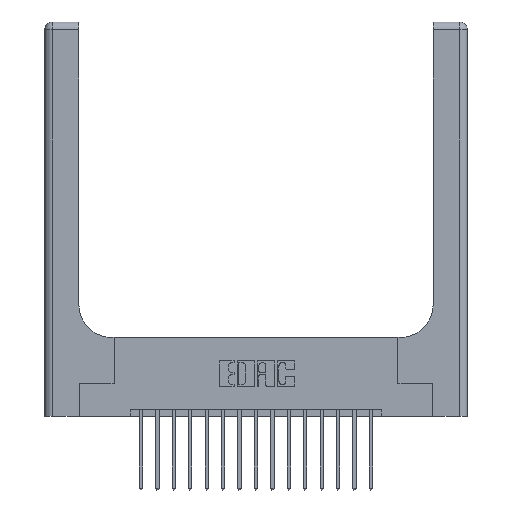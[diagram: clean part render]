
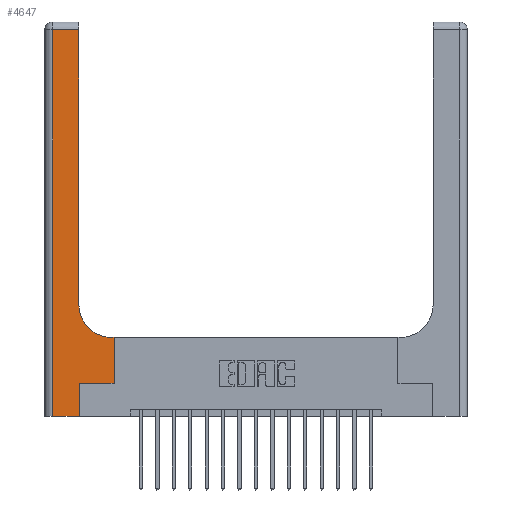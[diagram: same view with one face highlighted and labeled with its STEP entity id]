
A CAD part, top view. The second image highlights one B-rep face of the part: STEP entity #4647.
In plain terms, the highlighted planar face has unit normal (0, 0, 1).
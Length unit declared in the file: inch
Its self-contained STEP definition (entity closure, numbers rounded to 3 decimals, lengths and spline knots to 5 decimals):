
#137 = ORIENTED_EDGE ( 'NONE', *, *, #2642, .T. ) ;
#189 = PLANE ( 'NONE',  #9917 ) ;
#573 = VECTOR ( 'NONE', #8498, 39.37008 ) ;
#808 = VERTEX_POINT ( 'NONE', #2293 ) ;
#903 = CARTESIAN_POINT ( 'NONE',  ( 0.06, 0., 0.37 ) ) ;
#1154 = DIRECTION ( 'NONE',  ( -1., 0., 0. ) ) ;
#1228 = EDGE_CURVE ( 'NONE', #11090, #4433, #3883, .T. ) ;
#1326 = LINE ( 'NONE', #17534, #6257 ) ;
#1835 = DIRECTION ( 'NONE',  ( 0., 0., -1. ) ) ;
#1929 = CARTESIAN_POINT ( 'NONE',  ( 0., 3., 0.37 ) ) ;
#2078 = AXIS2_PLACEMENT_3D ( 'NONE', #3845, #6170, #7616 ) ;
#2280 = VERTEX_POINT ( 'NONE', #17408 ) ;
#2293 = CARTESIAN_POINT ( 'NONE',  ( 0.51, 0.6, 0.37 ) ) ;
#2421 = CARTESIAN_POINT ( 'NONE',  ( 0.26, 0.6, 0.37 ) ) ;
#2593 = VERTEX_POINT ( 'NONE', #903 ) ;
#2642 = EDGE_CURVE ( 'NONE', #6995, #12505, #8117, .T. ) ;
#2730 = EDGE_CURVE ( 'NONE', #2280, #17797, #15572, .T. ) ;
#3845 = CARTESIAN_POINT ( 'NONE',  ( 0.51, 0.85, 0.37 ) ) ;
#3883 = LINE ( 'NONE', #16996, #18015 ) ;
#4313 = DIRECTION ( 'NONE',  ( -1., 0., 0. ) ) ;
#4433 = VERTEX_POINT ( 'NONE', #9733 ) ;
#4647 = ADVANCED_FACE ( 'NONE', ( #6157 ), #189, .F. ) ;
#4959 = DIRECTION ( 'NONE',  ( 0., 1., 0. ) ) ;
#4995 = ORIENTED_EDGE ( 'NONE', *, *, #16987, .T. ) ;
#5085 = ORIENTED_EDGE ( 'NONE', *, *, #13222, .T. ) ;
#5392 = VECTOR ( 'NONE', #4959, 39.37008 ) ;
#5505 = DIRECTION ( 'NONE',  ( 0., 1., 0. ) ) ;
#5586 = VECTOR ( 'NONE', #18225, 39.37008 ) ;
#6157 = FACE_OUTER_BOUND ( 'NONE', #12662, .T. ) ;
#6170 = DIRECTION ( 'NONE',  ( 0., 0., -1. ) ) ;
#6257 = VECTOR ( 'NONE', #4313, 39.37008 ) ;
#6352 = VECTOR ( 'NONE', #10694, 39.37008 ) ;
#6433 = LINE ( 'NONE', #7973, #5586 ) ;
#6546 = CARTESIAN_POINT ( 'NONE',  ( 0.265, 0.25, 0.37 ) ) ;
#6584 = CARTESIAN_POINT ( 'NONE',  ( 0.528, 0.25, 0.37 ) ) ;
#6630 = EDGE_CURVE ( 'NONE', #4433, #808, #9903, .T. ) ;
#6811 = EDGE_CURVE ( 'NONE', #18609, #2593, #6433, .T. ) ;
#6967 = CARTESIAN_POINT ( 'NONE',  ( 0.265, 0., 0.37 ) ) ;
#6995 = VERTEX_POINT ( 'NONE', #17151 ) ;
#7407 = DIRECTION ( 'NONE',  ( -1., 0., 0. ) ) ;
#7616 = DIRECTION ( 'NONE',  ( 1., 0., 0. ) ) ;
#7907 = CIRCLE ( 'NONE', #2078, 0.25 ) ;
#7973 = CARTESIAN_POINT ( 'NONE',  ( 0.06, 3., 0.37 ) ) ;
#8117 = LINE ( 'NONE', #13922, #5392 ) ;
#8279 = CARTESIAN_POINT ( 'NONE',  ( 0., 0., 0.37 ) ) ;
#8498 = DIRECTION ( 'NONE',  ( 0., 1., 0. ) ) ;
#8754 = VECTOR ( 'NONE', #17072, 39.37008 ) ;
#9061 = ORIENTED_EDGE ( 'NONE', *, *, #18113, .T. ) ;
#9733 = CARTESIAN_POINT ( 'NONE',  ( 0.528, 0.6, 0.37 ) ) ;
#9903 = LINE ( 'NONE', #2421, #15764 ) ;
#9917 = AXIS2_PLACEMENT_3D ( 'NONE', #1929, #1835, #7407 ) ;
#10620 = CARTESIAN_POINT ( 'NONE',  ( 0.265, 0.25, 0.37 ) ) ;
#10694 = DIRECTION ( 'NONE',  ( 1., 0., 0. ) ) ;
#11090 = VERTEX_POINT ( 'NONE', #6584 ) ;
#11095 = ORIENTED_EDGE ( 'NONE', *, *, #15735, .T. ) ;
#12505 = VERTEX_POINT ( 'NONE', #15492 ) ;
#12662 = EDGE_LOOP ( 'NONE', ( #137, #11095, #15919, #4995, #16031, #9061, #13908, #14704, #5085 ) ) ;
#13222 = EDGE_CURVE ( 'NONE', #808, #6995, #7907, .T. ) ;
#13908 = ORIENTED_EDGE ( 'NONE', *, *, #1228, .T. ) ;
#13922 = CARTESIAN_POINT ( 'NONE',  ( 0.26, 3., 0.37 ) ) ;
#14077 = LINE ( 'NONE', #8279, #8754 ) ;
#14704 = ORIENTED_EDGE ( 'NONE', *, *, #6630, .T. ) ;
#15492 = CARTESIAN_POINT ( 'NONE',  ( 0.26, 2.94, 0.37 ) ) ;
#15572 = LINE ( 'NONE', #6967, #573 ) ;
#15735 = EDGE_CURVE ( 'NONE', #12505, #18609, #1326, .T. ) ;
#15764 = VECTOR ( 'NONE', #1154, 39.37008 ) ;
#15919 = ORIENTED_EDGE ( 'NONE', *, *, #6811, .T. ) ;
#16031 = ORIENTED_EDGE ( 'NONE', *, *, #2730, .T. ) ;
#16677 = CARTESIAN_POINT ( 'NONE',  ( 0.06, 2.94, 0.37 ) ) ;
#16884 = LINE ( 'NONE', #6546, #6352 ) ;
#16987 = EDGE_CURVE ( 'NONE', #2593, #2280, #14077, .T. ) ;
#16996 = CARTESIAN_POINT ( 'NONE',  ( 0.528, 0.25, 0.37 ) ) ;
#17072 = DIRECTION ( 'NONE',  ( 1., 0., 0. ) ) ;
#17151 = CARTESIAN_POINT ( 'NONE',  ( 0.26, 0.85, 0.37 ) ) ;
#17408 = CARTESIAN_POINT ( 'NONE',  ( 0.265, 0., 0.37 ) ) ;
#17534 = CARTESIAN_POINT ( 'NONE',  ( 0., 2.94, 0.37 ) ) ;
#17797 = VERTEX_POINT ( 'NONE', #10620 ) ;
#18015 = VECTOR ( 'NONE', #5505, 39.37008 ) ;
#18113 = EDGE_CURVE ( 'NONE', #17797, #11090, #16884, .T. ) ;
#18225 = DIRECTION ( 'NONE',  ( 0., -1., 0. ) ) ;
#18609 = VERTEX_POINT ( 'NONE', #16677 ) ;
